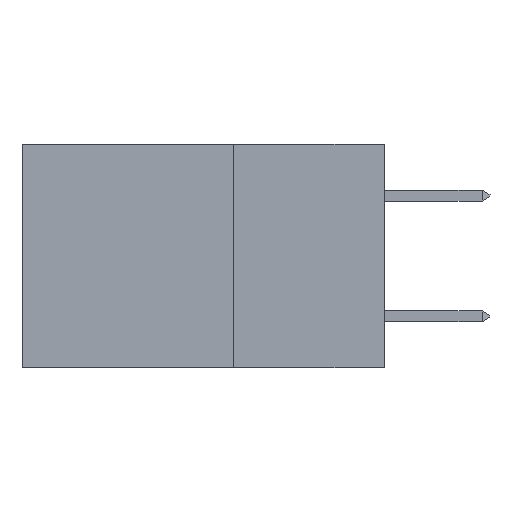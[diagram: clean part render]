
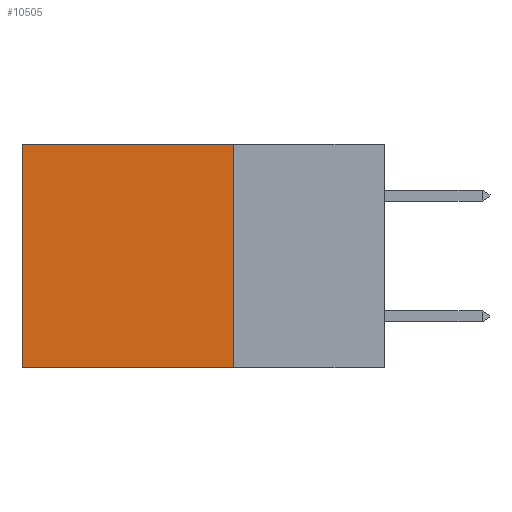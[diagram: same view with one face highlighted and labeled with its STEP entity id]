
A CAD part, left-side view. The second image highlights one B-rep face of the part: STEP entity #10505.
In plain terms, the highlighted planar face has unit normal (-1, 0, 0).
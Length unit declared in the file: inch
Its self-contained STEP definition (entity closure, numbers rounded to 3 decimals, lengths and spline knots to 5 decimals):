
#226 = CARTESIAN_POINT ( 'NONE',  ( 0.2875, 0.6, 0. ) ) ;
#1012 = EDGE_CURVE ( 'NONE', #8907, #1951, #3755, .T. ) ;
#1040 = EDGE_CURVE ( 'NONE', #4835, #10035, #2450, .T. ) ;
#1383 = VECTOR ( 'NONE', #3586, 39.37008 ) ;
#1439 = FACE_OUTER_BOUND ( 'NONE', #3082, .T. ) ;
#1507 = LINE ( 'NONE', #4425, #10165 ) ;
#1951 = VERTEX_POINT ( 'NONE', #3659 ) ;
#2450 = LINE ( 'NONE', #226, #1383 ) ;
#2515 = CARTESIAN_POINT ( 'NONE',  ( 0.2875, 0.25, 0. ) ) ;
#2734 = CARTESIAN_POINT ( 'NONE',  ( 0.2875, 0.6, 0. ) ) ;
#3082 = EDGE_LOOP ( 'NONE', ( #9876, #3690, #8509, #4440 ) ) ;
#3586 = DIRECTION ( 'NONE',  ( 0., 0., -1. ) ) ;
#3659 = CARTESIAN_POINT ( 'NONE',  ( 0.2875, 0.25, -0.37 ) ) ;
#3690 = ORIENTED_EDGE ( 'NONE', *, *, #8117, .F. ) ;
#3755 = LINE ( 'NONE', #2515, #3881 ) ;
#3843 = CARTESIAN_POINT ( 'NONE',  ( 0.2875, 0.25, 0. ) ) ;
#3881 = VECTOR ( 'NONE', #8437, 39.37008 ) ;
#3961 = PLANE ( 'NONE',  #5730 ) ;
#4425 = CARTESIAN_POINT ( 'NONE',  ( 0.2875, 0.25, -0.37 ) ) ;
#4440 = ORIENTED_EDGE ( 'NONE', *, *, #5914, .T. ) ;
#4835 = VERTEX_POINT ( 'NONE', #2734 ) ;
#5730 = AXIS2_PLACEMENT_3D ( 'NONE', #3843, #9736, #10588 ) ;
#5876 = CARTESIAN_POINT ( 'NONE',  ( 0.2875, 0.25, 0. ) ) ;
#5914 = EDGE_CURVE ( 'NONE', #8907, #4835, #8389, .T. ) ;
#6106 = DIRECTION ( 'NONE',  ( 0., 1., 0. ) ) ;
#6134 = VECTOR ( 'NONE', #10119, 39.37008 ) ;
#8117 = EDGE_CURVE ( 'NONE', #1951, #10035, #1507, .T. ) ;
#8389 = LINE ( 'NONE', #9286, #6134 ) ;
#8437 = DIRECTION ( 'NONE',  ( 0., 0., -1. ) ) ;
#8509 = ORIENTED_EDGE ( 'NONE', *, *, #1012, .F. ) ;
#8907 = VERTEX_POINT ( 'NONE', #5876 ) ;
#9286 = CARTESIAN_POINT ( 'NONE',  ( 0.2875, 0.25, 0. ) ) ;
#9736 = DIRECTION ( 'NONE',  ( 1., 0., 0. ) ) ;
#9876 = ORIENTED_EDGE ( 'NONE', *, *, #1040, .T. ) ;
#10035 = VERTEX_POINT ( 'NONE', #10072 ) ;
#10072 = CARTESIAN_POINT ( 'NONE',  ( 0.2875, 0.6, -0.37 ) ) ;
#10119 = DIRECTION ( 'NONE',  ( 0., 1., 0. ) ) ;
#10165 = VECTOR ( 'NONE', #6106, 39.37008 ) ;
#10505 = ADVANCED_FACE ( 'NONE', ( #1439 ), #3961, .F. ) ;
#10588 = DIRECTION ( 'NONE',  ( 0., 0., -1. ) ) ;
